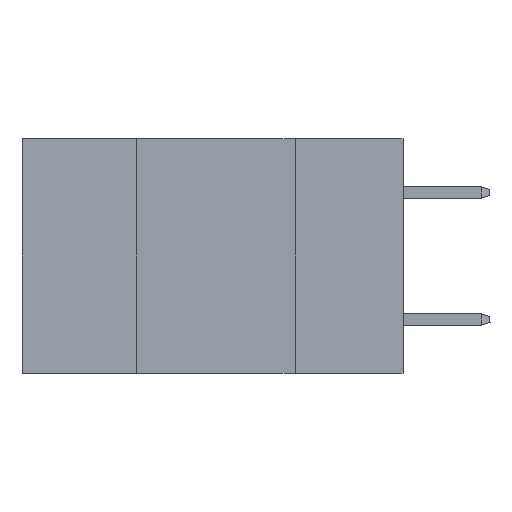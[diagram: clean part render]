
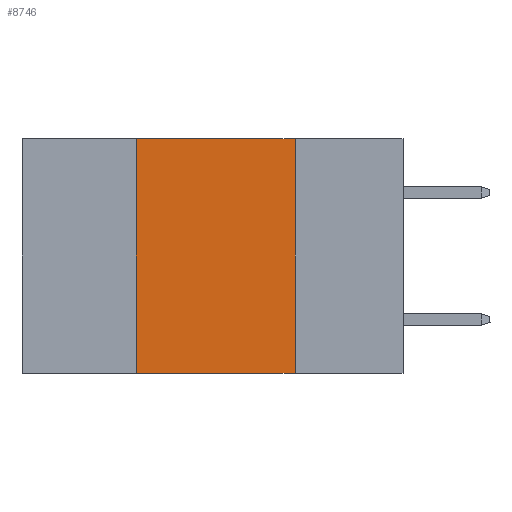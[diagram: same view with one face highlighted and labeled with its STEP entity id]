
A CAD part, left-side view. The second image highlights one B-rep face of the part: STEP entity #8746.
In plain terms, the highlighted planar face has unit normal (-1, 0, 0).
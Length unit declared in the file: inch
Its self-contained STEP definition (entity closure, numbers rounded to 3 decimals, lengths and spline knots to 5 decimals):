
#1452 = LINE ( 'NONE', #12037, #11810 ) ;
#1994 = CARTESIAN_POINT ( 'NONE',  ( 0., 0.6, -0.37 ) ) ;
#2277 = DIRECTION ( 'NONE',  ( 0., 0., -1. ) ) ;
#2358 = CARTESIAN_POINT ( 'NONE',  ( 0., 0.6, 0. ) ) ;
#2557 = ORIENTED_EDGE ( 'NONE', *, *, #8735, .F. ) ;
#2792 = DIRECTION ( 'NONE',  ( 0., 0., -1. ) ) ;
#2803 = ORIENTED_EDGE ( 'NONE', *, *, #8071, .F. ) ;
#3300 = ORIENTED_EDGE ( 'NONE', *, *, #3442, .F. ) ;
#3322 = EDGE_CURVE ( 'NONE', #9948, #13950, #11901, .T. ) ;
#3442 = EDGE_CURVE ( 'NONE', #9948, #14091, #1452, .T. ) ;
#4484 = FACE_OUTER_BOUND ( 'NONE', #7350, .T. ) ;
#5378 = CARTESIAN_POINT ( 'NONE',  ( 0., 0.17, -0.37 ) ) ;
#5890 = VECTOR ( 'NONE', #2792, 39.37008 ) ;
#5901 = DIRECTION ( 'NONE',  ( 0., 0., 1. ) ) ;
#6855 = CARTESIAN_POINT ( 'NONE',  ( 0., 0.42, 0. ) ) ;
#7151 = AXIS2_PLACEMENT_3D ( 'NONE', #8848, #12180, #2277 ) ;
#7350 = EDGE_LOOP ( 'NONE', ( #2803, #2557, #3300, #7622 ) ) ;
#7622 = ORIENTED_EDGE ( 'NONE', *, *, #3322, .T. ) ;
#8071 = EDGE_CURVE ( 'NONE', #13920, #13950, #13638, .T. ) ;
#8114 = CARTESIAN_POINT ( 'NONE',  ( 0., 0.17, 0. ) ) ;
#8735 = EDGE_CURVE ( 'NONE', #14091, #13920, #13362, .T. ) ;
#8746 = ADVANCED_FACE ( 'NONE', ( #4484 ), #11096, .F. ) ;
#8848 = CARTESIAN_POINT ( 'NONE',  ( 0., 0.6, 0. ) ) ;
#9948 = VERTEX_POINT ( 'NONE', #13035 ) ;
#10595 = VECTOR ( 'NONE', #12397, 39.37008 ) ;
#10898 = VECTOR ( 'NONE', #13081, 39.37008 ) ;
#11096 = PLANE ( 'NONE',  #7151 ) ;
#11810 = VECTOR ( 'NONE', #5901, 39.37008 ) ;
#11901 = LINE ( 'NONE', #1994, #10898 ) ;
#12037 = CARTESIAN_POINT ( 'NONE',  ( 0., 0.42, 0. ) ) ;
#12180 = DIRECTION ( 'NONE',  ( 1., 0., 0. ) ) ;
#12397 = DIRECTION ( 'NONE',  ( 0., -1., 0. ) ) ;
#13035 = CARTESIAN_POINT ( 'NONE',  ( 0., 0.42, -0.37 ) ) ;
#13081 = DIRECTION ( 'NONE',  ( 0., -1., 0. ) ) ;
#13159 = CARTESIAN_POINT ( 'NONE',  ( 0., 0.17, 0. ) ) ;
#13362 = LINE ( 'NONE', #2358, #10595 ) ;
#13638 = LINE ( 'NONE', #8114, #5890 ) ;
#13920 = VERTEX_POINT ( 'NONE', #13159 ) ;
#13950 = VERTEX_POINT ( 'NONE', #5378 ) ;
#14091 = VERTEX_POINT ( 'NONE', #6855 ) ;
